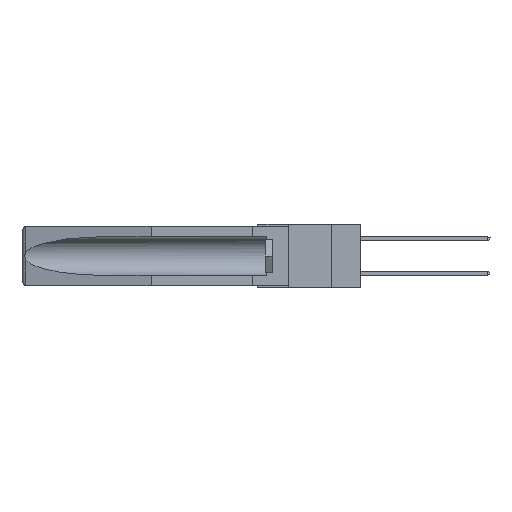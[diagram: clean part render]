
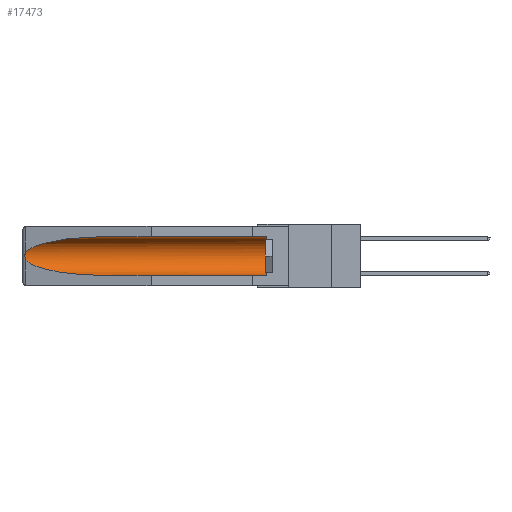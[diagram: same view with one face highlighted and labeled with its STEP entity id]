
A CAD part, left-side view. The second image highlights one B-rep face of the part: STEP entity #17473.
In plain terms, the highlighted cylindrical face has radius 2.857 mm (diameter 5.715 mm), a partial arc.
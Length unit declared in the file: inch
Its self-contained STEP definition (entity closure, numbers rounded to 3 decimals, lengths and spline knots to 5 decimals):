
#951 = CARTESIAN_POINT ( 'NONE',  ( 0.26597, 1.52961, -0.15275 ) ) ;
#1410 = DIRECTION ( 'NONE',  ( 0., 0., 1. ) ) ;
#2965 = CARTESIAN_POINT ( 'NONE',  ( 0.25451, 1.48313, -0.24835 ) ) ;
#3175 = VERTEX_POINT ( 'NONE', #4128 ) ;
#3536 = FACE_OUTER_BOUND ( 'NONE', #18433, .T. ) ;
#3540 = CARTESIAN_POINT ( 'NONE',  ( 0.26537, 1.52718, -0.14972 ) ) ;
#4031 = CARTESIAN_POINT ( 'NONE',  ( 0.155, -0.30754, -0.059 ) ) ;
#4128 = CARTESIAN_POINT ( 'NONE',  ( 0.155, 0.126, -0.284 ) ) ;
#4499 = DIRECTION ( 'NONE',  ( 0., 0., 1. ) ) ;
#5082 = VERTEX_POINT ( 'NONE', #6912 ) ;
#5126 = EDGE_CURVE ( 'NONE', #3175, #11340, #12641, .T. ) ;
#5646 = CARTESIAN_POINT ( 'NONE',  ( 0.21114, 1.30732, -0.284 ) ) ;
#6912 = CARTESIAN_POINT ( 'NONE',  ( 0.26537, 1.52718, -0.19328 ) ) ;
#7214 = VERTEX_POINT ( 'NONE', #3540 ) ;
#7384 = ORIENTED_EDGE ( 'NONE', *, *, #15459, .T. ) ;
#7511 = CARTESIAN_POINT ( 'NONE',  ( 0.26537, 1.52718, -0.19328 ) ) ;
#7574 = VERTEX_POINT ( 'NONE', #17065 ) ;
#8303 = CYLINDRICAL_SURFACE ( 'NONE', #19024, 0.1125 ) ;
#9139 = CARTESIAN_POINT ( 'NONE',  ( 0.26537, 1.52718, -0.19328 ) ) ;
#9833 = VECTOR ( 'NONE', #16253, 39.37008 ) ;
#9860 = AXIS2_PLACEMENT_3D ( 'NONE', #10648, #13529, #4499 ) ;
#9867 = B_SPLINE_CURVE_WITH_KNOTS ( 'NONE', 3,
 ( #10062, #951, #9999, #11576, #13070, #16778, #15321, #19621, #10633, #9139 ),
 .UNSPECIFIED., .F., .F.,
 ( 4, 2, 2, 2, 4 ),
 ( 0., 0.00029, 0.00058, 0.00087, 0.00117 ),
 .UNSPECIFIED. ) ;
#9999 = CARTESIAN_POINT ( 'NONE',  ( 0.26654, 1.53092, -0.15636 ) ) ;
#10062 = CARTESIAN_POINT ( 'NONE',  ( 0.26537, 1.52718, -0.14972 ) ) ;
#10165 = CARTESIAN_POINT ( 'NONE',  ( 0.155, -0.30754, -0.284 ) ) ;
#10593 = DIRECTION ( 'NONE',  ( 0., 1., 0. ) ) ;
#10633 = CARTESIAN_POINT ( 'NONE',  ( 0.26597, 1.5296, -0.19026 ) ) ;
#10648 = CARTESIAN_POINT ( 'NONE',  ( 0.155, 0.126, -0.1715 ) ) ;
#10880 = VERTEX_POINT ( 'NONE', #18717 ) ;
#11311 =( BOUNDED_CURVE ( )  B_SPLINE_CURVE ( 3, ( #17618, #13162, #17964, #14743 ),
 .UNSPECIFIED., .F., .F. ) 
 B_SPLINE_CURVE_WITH_KNOTS ( ( 4, 4 ),
 ( 4.71239, 6.08839 ),
 .UNSPECIFIED. ) 
 CURVE ( )  GEOMETRIC_REPRESENTATION_ITEM ( )  RATIONAL_B_SPLINE_CURVE ( ( 1., 0.848, 0.848, 1. ) ) 
 REPRESENTATION_ITEM ( '' )  );
#11340 = VERTEX_POINT ( 'NONE', #13717 ) ;
#11576 = CARTESIAN_POINT ( 'NONE',  ( 0.2673, 1.5327, -0.16383 ) ) ;
#11590 = CARTESIAN_POINT ( 'NONE',  ( 0.155, 1.07973, -0.284 ) ) ;
#12067 = VECTOR ( 'NONE', #17658, 39.37008 ) ;
#12641 = LINE ( 'NONE', #10165, #9833 ) ;
#13070 = CARTESIAN_POINT ( 'NONE',  ( 0.2675, 1.53308, -0.16763 ) ) ;
#13162 = CARTESIAN_POINT ( 'NONE',  ( 0.21114, 1.30732, -0.059 ) ) ;
#13529 = DIRECTION ( 'NONE',  ( 0., -1., 0. ) ) ;
#13717 = CARTESIAN_POINT ( 'NONE',  ( 0.155, 1.07973, -0.284 ) ) ;
#14187 = ORIENTED_EDGE ( 'NONE', *, *, #17368, .T. ) ;
#14518 = ORIENTED_EDGE ( 'NONE', *, *, #18708, .T. ) ;
#14743 = CARTESIAN_POINT ( 'NONE',  ( 0.26537, 1.52718, -0.14972 ) ) ;
#14991 = CIRCLE ( 'NONE', #9860, 0.1125 ) ;
#15321 = CARTESIAN_POINT ( 'NONE',  ( 0.2673, 1.53269, -0.17917 ) ) ;
#15341 = ORIENTED_EDGE ( 'NONE', *, *, #19324, .T. ) ;
#15459 = EDGE_CURVE ( 'NONE', #3175, #10880, #14991, .T. ) ;
#16253 = DIRECTION ( 'NONE',  ( 0., 1., 0. ) ) ;
#16510 = EDGE_CURVE ( 'NONE', #5082, #11340, #17495, .T. ) ;
#16778 = CARTESIAN_POINT ( 'NONE',  ( 0.2675, 1.53308, -0.17534 ) ) ;
#17065 = CARTESIAN_POINT ( 'NONE',  ( 0.155, 1.07973, -0.059 ) ) ;
#17368 = EDGE_CURVE ( 'NONE', #10880, #7574, #19642, .T. ) ;
#17473 = ADVANCED_FACE ( 'NONE', ( #3536 ), #8303, .F. ) ;
#17495 =( BOUNDED_CURVE ( )  B_SPLINE_CURVE ( 3, ( #7511, #2965, #5646, #11590 ),
 .UNSPECIFIED., .F., .F. ) 
 B_SPLINE_CURVE_WITH_KNOTS ( ( 4, 4 ),
 ( 0.1948, 1.5708 ),
 .UNSPECIFIED. ) 
 CURVE ( )  GEOMETRIC_REPRESENTATION_ITEM ( )  RATIONAL_B_SPLINE_CURVE ( ( 1., 0.848, 0.848, 1. ) ) 
 REPRESENTATION_ITEM ( '' )  );
#17618 = CARTESIAN_POINT ( 'NONE',  ( 0.155, 1.07973, -0.059 ) ) ;
#17658 = DIRECTION ( 'NONE',  ( 0., 1., 0. ) ) ;
#17964 = CARTESIAN_POINT ( 'NONE',  ( 0.25451, 1.48313, -0.09465 ) ) ;
#18001 = CARTESIAN_POINT ( 'NONE',  ( 0.155, -0.30754, -0.1715 ) ) ;
#18140 = ORIENTED_EDGE ( 'NONE', *, *, #16510, .T. ) ;
#18433 = EDGE_LOOP ( 'NONE', ( #15341, #14518, #18140, #18489, #7384, #14187 ) ) ;
#18489 = ORIENTED_EDGE ( 'NONE', *, *, #5126, .F. ) ;
#18708 = EDGE_CURVE ( 'NONE', #7214, #5082, #9867, .T. ) ;
#18717 = CARTESIAN_POINT ( 'NONE',  ( 0.155, 0.126, -0.059 ) ) ;
#19024 = AXIS2_PLACEMENT_3D ( 'NONE', #18001, #10593, #1410 ) ;
#19324 = EDGE_CURVE ( 'NONE', #7574, #7214, #11311, .T. ) ;
#19621 = CARTESIAN_POINT ( 'NONE',  ( 0.26655, 1.53094, -0.18657 ) ) ;
#19642 = LINE ( 'NONE', #4031, #12067 ) ;
